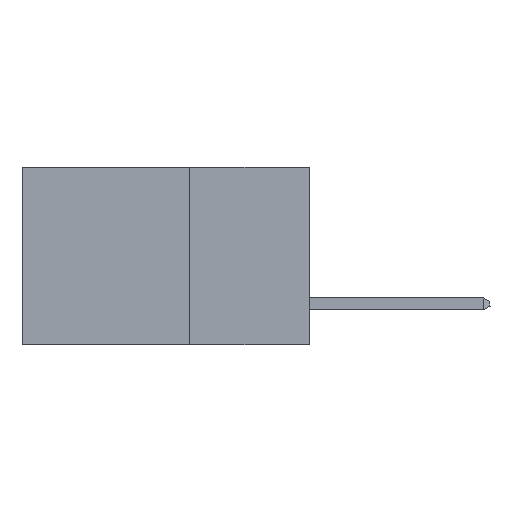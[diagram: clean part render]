
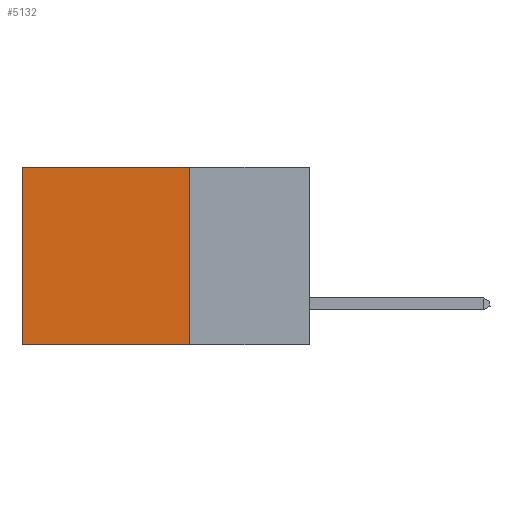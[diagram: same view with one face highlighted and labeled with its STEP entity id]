
A CAD part, left-side view. The second image highlights one B-rep face of the part: STEP entity #5132.
In plain terms, the highlighted planar face has unit normal (-1, 0, 0).
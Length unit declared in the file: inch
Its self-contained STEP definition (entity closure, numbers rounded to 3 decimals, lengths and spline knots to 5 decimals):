
#29 = DIRECTION ( 'NONE',  ( 1., 0., 0. ) ) ;
#1106 = DIRECTION ( 'NONE',  ( 0., 1., 0. ) ) ;
#1989 = ORIENTED_EDGE ( 'NONE', *, *, #24703, .F. ) ;
#2597 = ORIENTED_EDGE ( 'NONE', *, *, #14420, .T. ) ;
#4702 = VERTEX_POINT ( 'NONE', #22053 ) ;
#4756 = EDGE_CURVE ( 'NONE', #12705, #4702, #7220, .T. ) ;
#5132 = ADVANCED_FACE ( 'NONE', ( #9450 ), #7280, .F. ) ;
#5362 = ORIENTED_EDGE ( 'NONE', *, *, #30551, .F. ) ;
#6545 = LINE ( 'NONE', #18220, #8051 ) ;
#6672 = ORIENTED_EDGE ( 'NONE', *, *, #4756, .T. ) ;
#7220 = LINE ( 'NONE', #29317, #10247 ) ;
#7280 = PLANE ( 'NONE',  #27326 ) ;
#7538 = CARTESIAN_POINT ( 'NONE',  ( 0.2875, 0.25, 0. ) ) ;
#7583 = DIRECTION ( 'NONE',  ( 0., 0., -1. ) ) ;
#8051 = VECTOR ( 'NONE', #1106, 39.37008 ) ;
#9450 = FACE_OUTER_BOUND ( 'NONE', #11450, .T. ) ;
#9608 = LINE ( 'NONE', #7538, #30989 ) ;
#10247 = VECTOR ( 'NONE', #7583, 39.37008 ) ;
#11450 = EDGE_LOOP ( 'NONE', ( #6672, #5362, #1989, #2597 ) ) ;
#12705 = VERTEX_POINT ( 'NONE', #30851 ) ;
#12753 = DIRECTION ( 'NONE',  ( 0., 0., -1. ) ) ;
#12810 = LINE ( 'NONE', #13114, #22304 ) ;
#13114 = CARTESIAN_POINT ( 'NONE',  ( 0.2875, 0.25, 0. ) ) ;
#13422 = VERTEX_POINT ( 'NONE', #27185 ) ;
#14420 = EDGE_CURVE ( 'NONE', #13422, #12705, #12810, .T. ) ;
#17502 = CARTESIAN_POINT ( 'NONE',  ( 0.2875, 0.25, -0.37 ) ) ;
#18220 = CARTESIAN_POINT ( 'NONE',  ( 0.2875, 0.25, -0.37 ) ) ;
#22053 = CARTESIAN_POINT ( 'NONE',  ( 0.2875, 0.6, -0.37 ) ) ;
#22304 = VECTOR ( 'NONE', #25416, 39.37008 ) ;
#24279 = CARTESIAN_POINT ( 'NONE',  ( 0.2875, 0.25, 0. ) ) ;
#24362 = VERTEX_POINT ( 'NONE', #17502 ) ;
#24703 = EDGE_CURVE ( 'NONE', #13422, #24362, #9608, .T. ) ;
#24889 = DIRECTION ( 'NONE',  ( 0., 0., -1. ) ) ;
#25416 = DIRECTION ( 'NONE',  ( 0., 1., 0. ) ) ;
#27185 = CARTESIAN_POINT ( 'NONE',  ( 0.2875, 0.25, 0. ) ) ;
#27326 = AXIS2_PLACEMENT_3D ( 'NONE', #24279, #29, #24889 ) ;
#29317 = CARTESIAN_POINT ( 'NONE',  ( 0.2875, 0.6, 0. ) ) ;
#30551 = EDGE_CURVE ( 'NONE', #24362, #4702, #6545, .T. ) ;
#30851 = CARTESIAN_POINT ( 'NONE',  ( 0.2875, 0.6, 0. ) ) ;
#30989 = VECTOR ( 'NONE', #12753, 39.37008 ) ;
